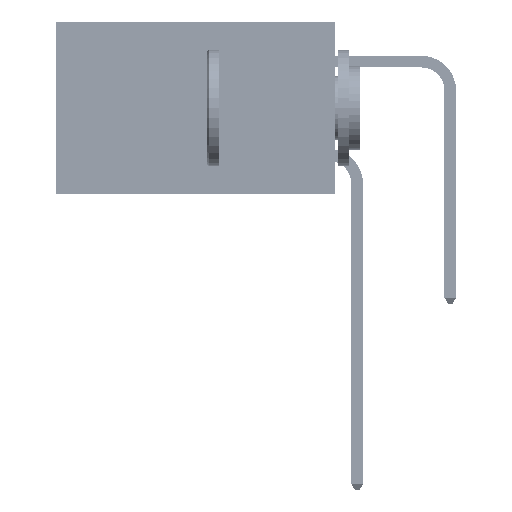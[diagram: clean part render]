
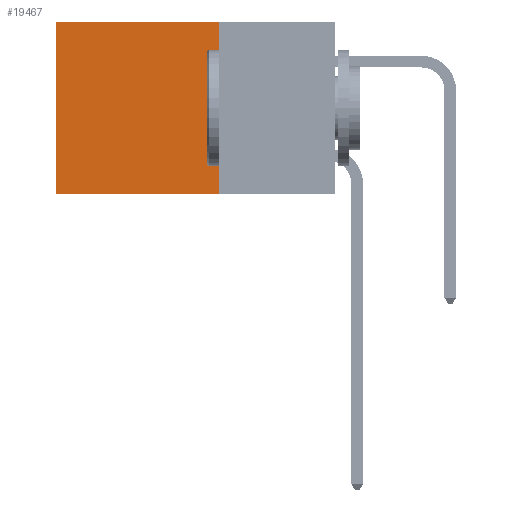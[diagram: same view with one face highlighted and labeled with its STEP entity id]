
A CAD part, left-side view. The second image highlights one B-rep face of the part: STEP entity #19467.
In plain terms, the highlighted planar face has unit normal (-1, 0, 0).
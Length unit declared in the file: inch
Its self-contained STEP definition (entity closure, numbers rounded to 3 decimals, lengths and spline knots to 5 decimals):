
#285 = VECTOR ( 'NONE', #39505, 39.37008 ) ;
#2067 = VECTOR ( 'NONE', #2753, 39.37008 ) ;
#2294 = VECTOR ( 'NONE', #28639, 39.37008 ) ;
#2753 = DIRECTION ( 'NONE',  ( 0., 1., 0. ) ) ;
#6211 = FACE_OUTER_BOUND ( 'NONE', #38666, .T. ) ;
#7613 = ORIENTED_EDGE ( 'NONE', *, *, #27654, .F. ) ;
#9880 = CARTESIAN_POINT ( 'NONE',  ( 0.2875, 0.25, 0. ) ) ;
#10563 = VERTEX_POINT ( 'NONE', #9880 ) ;
#11406 = ORIENTED_EDGE ( 'NONE', *, *, #25160, .F. ) ;
#11495 = CARTESIAN_POINT ( 'NONE',  ( 0.2875, 0.6, 0. ) ) ;
#12221 = LINE ( 'NONE', #29248, #2067 ) ;
#19467 = ADVANCED_FACE ( 'NONE', ( #6211 ), #20303, .F. ) ;
#20303 = PLANE ( 'NONE',  #44667 ) ;
#20477 = VERTEX_POINT ( 'NONE', #43201 ) ;
#20584 = LINE ( 'NONE', #35719, #285 ) ;
#21198 = EDGE_CURVE ( 'NONE', #10563, #46664, #20584, .T. ) ;
#23419 = CARTESIAN_POINT ( 'NONE',  ( 0.2875, 0.6, -0.37 ) ) ;
#24066 = DIRECTION ( 'NONE',  ( 0., 0., -1. ) ) ;
#24859 = CARTESIAN_POINT ( 'NONE',  ( 0.2875, 0.25, 0. ) ) ;
#24926 = VERTEX_POINT ( 'NONE', #23419 ) ;
#25160 = EDGE_CURVE ( 'NONE', #10563, #20477, #42538, .T. ) ;
#26056 = VECTOR ( 'NONE', #41659, 39.37008 ) ;
#27654 = EDGE_CURVE ( 'NONE', #20477, #24926, #12221, .T. ) ;
#28435 = LINE ( 'NONE', #11495, #26056 ) ;
#28639 = DIRECTION ( 'NONE',  ( 0., 0., -1. ) ) ;
#29122 = ORIENTED_EDGE ( 'NONE', *, *, #34904, .T. ) ;
#29248 = CARTESIAN_POINT ( 'NONE',  ( 0.2875, 0.25, -0.37 ) ) ;
#31459 = CARTESIAN_POINT ( 'NONE',  ( 0.2875, 0.25, 0. ) ) ;
#34904 = EDGE_CURVE ( 'NONE', #46664, #24926, #28435, .T. ) ;
#35719 = CARTESIAN_POINT ( 'NONE',  ( 0.2875, 0.25, 0. ) ) ;
#38666 = EDGE_LOOP ( 'NONE', ( #29122, #7613, #11406, #42652 ) ) ;
#39505 = DIRECTION ( 'NONE',  ( 0., 1., 0. ) ) ;
#41659 = DIRECTION ( 'NONE',  ( 0., 0., -1. ) ) ;
#42538 = LINE ( 'NONE', #24859, #2294 ) ;
#42652 = ORIENTED_EDGE ( 'NONE', *, *, #21198, .T. ) ;
#43201 = CARTESIAN_POINT ( 'NONE',  ( 0.2875, 0.25, -0.37 ) ) ;
#44667 = AXIS2_PLACEMENT_3D ( 'NONE', #31459, #46579, #24066 ) ;
#45304 = CARTESIAN_POINT ( 'NONE',  ( 0.2875, 0.6, 0. ) ) ;
#46579 = DIRECTION ( 'NONE',  ( 1., 0., 0. ) ) ;
#46664 = VERTEX_POINT ( 'NONE', #45304 ) ;
